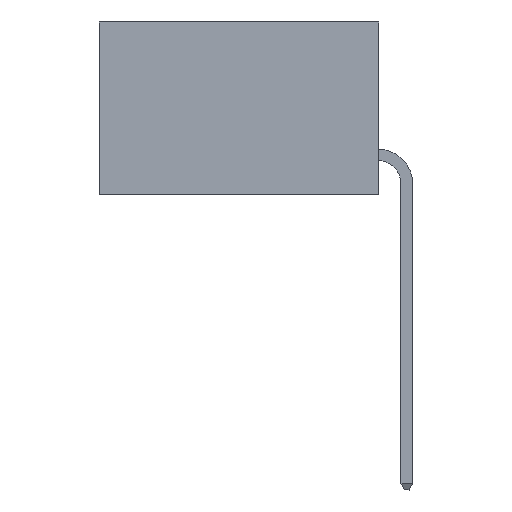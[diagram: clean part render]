
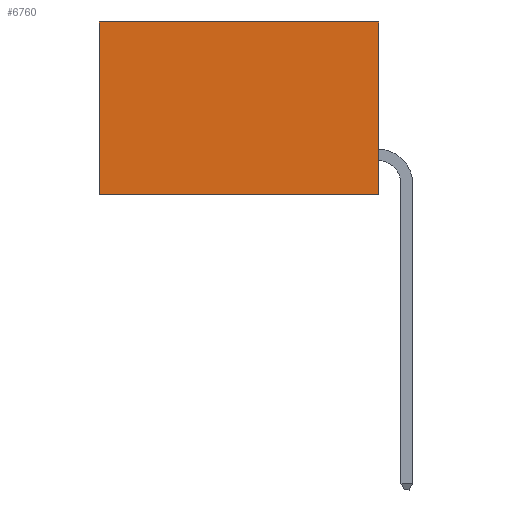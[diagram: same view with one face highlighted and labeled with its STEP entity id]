
A CAD part, left-side view. The second image highlights one B-rep face of the part: STEP entity #6760.
In plain terms, the highlighted planar face has unit normal (-1, 0, 0).
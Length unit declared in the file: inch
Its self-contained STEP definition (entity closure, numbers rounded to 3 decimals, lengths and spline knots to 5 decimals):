
#490 = EDGE_CURVE ( 'NONE', #6070, #12586, #8551, .T. ) ;
#650 = VECTOR ( 'NONE', #14298, 39.37008 ) ;
#808 = ORIENTED_EDGE ( 'NONE', *, *, #10277, .F. ) ;
#1341 = CARTESIAN_POINT ( 'NONE',  ( 0.2615, 0., -0.37 ) ) ;
#2487 = PLANE ( 'NONE',  #5307 ) ;
#3168 = EDGE_CURVE ( 'NONE', #13623, #6070, #8962, .T. ) ;
#4432 = DIRECTION ( 'NONE',  ( 0., 0., -1. ) ) ;
#5307 = AXIS2_PLACEMENT_3D ( 'NONE', #1341, #13639, #4432 ) ;
#5619 = ORIENTED_EDGE ( 'NONE', *, *, #3168, .T. ) ;
#5946 = DIRECTION ( 'NONE',  ( 0., 0., -1. ) ) ;
#6037 = VECTOR ( 'NONE', #10309, 39.37008 ) ;
#6070 = VERTEX_POINT ( 'NONE', #10789 ) ;
#6760 = ADVANCED_FACE ( 'NONE', ( #12802 ), #2487, .F. ) ;
#7771 = DIRECTION ( 'NONE',  ( 0., 1., 0. ) ) ;
#7916 = CARTESIAN_POINT ( 'NONE',  ( 0.2615, 0., -0.37 ) ) ;
#8017 = CARTESIAN_POINT ( 'NONE',  ( 0.2615, 0., 0. ) ) ;
#8551 = LINE ( 'NONE', #9680, #650 ) ;
#8962 = LINE ( 'NONE', #9024, #10784 ) ;
#9024 = CARTESIAN_POINT ( 'NONE',  ( 0.2615, 0., 0. ) ) ;
#9680 = CARTESIAN_POINT ( 'NONE',  ( 0.2615, 0.6, -0.37 ) ) ;
#10097 = CARTESIAN_POINT ( 'NONE',  ( 0.2615, 0., -0.37 ) ) ;
#10277 = EDGE_CURVE ( 'NONE', #13243, #12586, #13649, .T. ) ;
#10309 = DIRECTION ( 'NONE',  ( 0., 1., 0. ) ) ;
#10784 = VECTOR ( 'NONE', #7771, 39.37008 ) ;
#10789 = CARTESIAN_POINT ( 'NONE',  ( 0.2615, 0.6, 0. ) ) ;
#10987 = VECTOR ( 'NONE', #5946, 39.37008 ) ;
#11708 = CARTESIAN_POINT ( 'NONE',  ( 0.2615, 0.6, -0.37 ) ) ;
#12100 = EDGE_CURVE ( 'NONE', #13623, #13243, #13095, .T. ) ;
#12409 = ORIENTED_EDGE ( 'NONE', *, *, #12100, .F. ) ;
#12586 = VERTEX_POINT ( 'NONE', #11708 ) ;
#12802 = FACE_OUTER_BOUND ( 'NONE', #14314, .T. ) ;
#12868 = CARTESIAN_POINT ( 'NONE',  ( 0.2615, 0., -0.37 ) ) ;
#13095 = LINE ( 'NONE', #12868, #10987 ) ;
#13243 = VERTEX_POINT ( 'NONE', #10097 ) ;
#13500 = ORIENTED_EDGE ( 'NONE', *, *, #490, .T. ) ;
#13623 = VERTEX_POINT ( 'NONE', #8017 ) ;
#13639 = DIRECTION ( 'NONE',  ( 1., 0., 0. ) ) ;
#13649 = LINE ( 'NONE', #7916, #6037 ) ;
#14298 = DIRECTION ( 'NONE',  ( 0., 0., -1. ) ) ;
#14314 = EDGE_LOOP ( 'NONE', ( #13500, #808, #12409, #5619 ) ) ;
